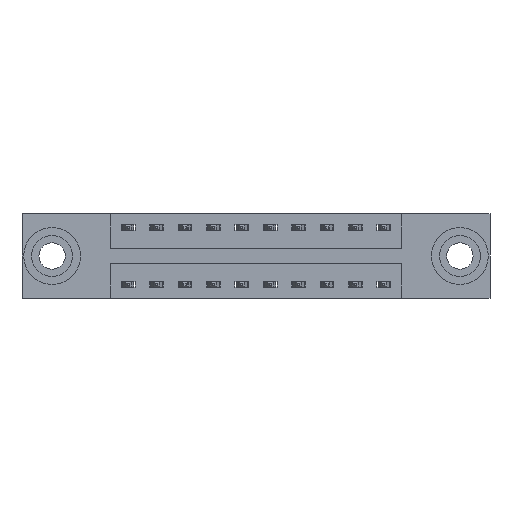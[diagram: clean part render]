
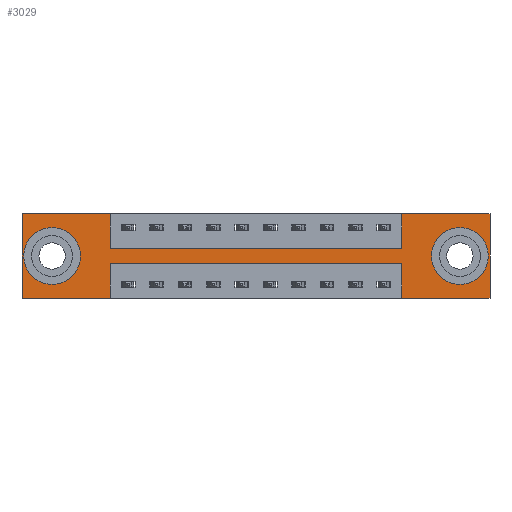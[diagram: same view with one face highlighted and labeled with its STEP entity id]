
A CAD part, front view. The second image highlights one B-rep face of the part: STEP entity #3029.
In plain terms, the highlighted planar face has unit normal (0, -1, 0).
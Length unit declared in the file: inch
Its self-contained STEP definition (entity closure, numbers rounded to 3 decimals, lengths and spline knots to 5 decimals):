
#283 = DIRECTION ( 'NONE',  ( 0., 0., -1. ) ) ;
#400 = DIRECTION ( 'NONE',  ( -1., 0., 0. ) ) ;
#418 = VERTEX_POINT ( 'NONE', #2137 ) ;
#450 = DIRECTION ( 'NONE',  ( 0., -1., 0. ) ) ;
#563 = VECTOR ( 'NONE', #8137, 39.37008 ) ;
#640 = CARTESIAN_POINT ( 'NONE',  ( 0., 0., -0.37 ) ) ;
#755 = LINE ( 'NONE', #9937, #563 ) ;
#928 = CARTESIAN_POINT ( 'NONE',  ( 0.1325, 0., -0.185 ) ) ;
#998 = ORIENTED_EDGE ( 'NONE', *, *, #1817, .F. ) ;
#1020 = ORIENTED_EDGE ( 'NONE', *, *, #8218, .F. ) ;
#1084 = ORIENTED_EDGE ( 'NONE', *, *, #1894, .F. ) ;
#1175 = VERTEX_POINT ( 'NONE', #8202 ) ;
#1240 = VERTEX_POINT ( 'NONE', #2220 ) ;
#1372 = EDGE_CURVE ( 'NONE', #11254, #5622, #755, .T. ) ;
#1417 = CARTESIAN_POINT ( 'NONE',  ( 0., 0., -0.37 ) ) ;
#1468 = DIRECTION ( 'NONE',  ( 1., 0., 0. ) ) ;
#1470 = CARTESIAN_POINT ( 'NONE',  ( 0., 0., -0.37 ) ) ;
#1503 = CARTESIAN_POINT ( 'NONE',  ( 0.1325, 0., -0.263 ) ) ;
#1510 = LINE ( 'NONE', #11668, #4019 ) ;
#1596 = EDGE_CURVE ( 'NONE', #10452, #1175, #2704, .T. ) ;
#1668 = CARTESIAN_POINT ( 'NONE',  ( 0., 0., 0. ) ) ;
#1709 = EDGE_LOOP ( 'NONE', ( #7760, #5570, #1020, #5582, #10190, #3095, #998, #7753, #9215, #1084, #11849, #6446 ) ) ;
#1753 = EDGE_CURVE ( 'NONE', #418, #9596, #5391, .T. ) ;
#1760 = CIRCLE ( 'NONE', #7940, 0.078 ) ;
#1817 = EDGE_CURVE ( 'NONE', #11834, #3620, #11511, .T. ) ;
#1894 = EDGE_CURVE ( 'NONE', #10943, #7213, #6140, .T. ) ;
#1963 = DIRECTION ( 'NONE',  ( 0., 0., 1. ) ) ;
#2026 = FACE_BOUND ( 'NONE', #10474, .T. ) ;
#2090 = CARTESIAN_POINT ( 'NONE',  ( 0., 0., 0. ) ) ;
#2137 = CARTESIAN_POINT ( 'NONE',  ( 1.9275, 0., -0.263 ) ) ;
#2142 = EDGE_CURVE ( 'NONE', #1240, #11254, #7917, .T. ) ;
#2166 = CARTESIAN_POINT ( 'NONE',  ( 1.6725, 0., -0.37 ) ) ;
#2220 = CARTESIAN_POINT ( 'NONE',  ( 1.6725, 0., -0.22 ) ) ;
#2416 = DIRECTION ( 'NONE',  ( 0., 1., 0. ) ) ;
#2452 = ORIENTED_EDGE ( 'NONE', *, *, #1753, .T. ) ;
#2470 = LINE ( 'NONE', #640, #4967 ) ;
#2604 = VERTEX_POINT ( 'NONE', #2166 ) ;
#2684 = VECTOR ( 'NONE', #8916, 39.37008 ) ;
#2704 = CIRCLE ( 'NONE', #7905, 0.078 ) ;
#2754 = EDGE_LOOP ( 'NONE', ( #5229, #2785 ) ) ;
#2785 = ORIENTED_EDGE ( 'NONE', *, *, #1596, .T. ) ;
#2808 = EDGE_CURVE ( 'NONE', #1175, #10452, #1760, .T. ) ;
#2999 = VERTEX_POINT ( 'NONE', #8491 ) ;
#3029 = ADVANCED_FACE ( 'NONE', ( #2026, #4878, #5725 ), #9387, .T. ) ;
#3070 = VECTOR ( 'NONE', #1468, 39.37008 ) ;
#3093 = DIRECTION ( 'NONE',  ( 1., 0., 0. ) ) ;
#3095 = ORIENTED_EDGE ( 'NONE', *, *, #10859, .F. ) ;
#3135 = DIRECTION ( 'NONE',  ( 0., 0., -1. ) ) ;
#3156 = EDGE_CURVE ( 'NONE', #5622, #8309, #3539, .T. ) ;
#3242 = DIRECTION ( 'NONE',  ( 0., 0., 1. ) ) ;
#3278 = VECTOR ( 'NONE', #7834, 39.37008 ) ;
#3320 = DIRECTION ( 'NONE',  ( 0., 0., 1. ) ) ;
#3539 = LINE ( 'NONE', #1470, #5500 ) ;
#3620 = VERTEX_POINT ( 'NONE', #11077 ) ;
#3794 = CARTESIAN_POINT ( 'NONE',  ( 0.3875, 0., 0. ) ) ;
#4019 = VECTOR ( 'NONE', #4307, 39.37008 ) ;
#4117 = LINE ( 'NONE', #11361, #5005 ) ;
#4129 = VECTOR ( 'NONE', #7740, 39.37008 ) ;
#4212 = DIRECTION ( 'NONE',  ( 0., 1., 0. ) ) ;
#4229 = CARTESIAN_POINT ( 'NONE',  ( 2.06, 0., 0. ) ) ;
#4307 = DIRECTION ( 'NONE',  ( 1., 0., 0. ) ) ;
#4337 = CARTESIAN_POINT ( 'NONE',  ( 0.1325, 0., -0.185 ) ) ;
#4403 = LINE ( 'NONE', #5307, #2684 ) ;
#4490 = ORIENTED_EDGE ( 'NONE', *, *, #4623, .T. ) ;
#4623 = EDGE_CURVE ( 'NONE', #9596, #418, #6674, .T. ) ;
#4627 = DIRECTION ( 'NONE',  ( 0., 1., 0. ) ) ;
#4681 = DIRECTION ( 'NONE',  ( 0., 0., -1. ) ) ;
#4878 = FACE_BOUND ( 'NONE', #2754, .T. ) ;
#4967 = VECTOR ( 'NONE', #400, 39.37008 ) ;
#5005 = VECTOR ( 'NONE', #3093, 39.37008 ) ;
#5229 = ORIENTED_EDGE ( 'NONE', *, *, #2808, .T. ) ;
#5252 = CARTESIAN_POINT ( 'NONE',  ( 1.9275, 0., -0.107 ) ) ;
#5307 = CARTESIAN_POINT ( 'NONE',  ( 2.06, 0., 0. ) ) ;
#5391 = CIRCLE ( 'NONE', #11591, 0.078 ) ;
#5478 = CARTESIAN_POINT ( 'NONE',  ( 1.9275, 0., -0.185 ) ) ;
#5500 = VECTOR ( 'NONE', #10606, 39.37008 ) ;
#5553 = VECTOR ( 'NONE', #1963, 39.37008 ) ;
#5570 = ORIENTED_EDGE ( 'NONE', *, *, #2142, .F. ) ;
#5582 = ORIENTED_EDGE ( 'NONE', *, *, #6201, .F. ) ;
#5622 = VERTEX_POINT ( 'NONE', #7486 ) ;
#5725 = FACE_OUTER_BOUND ( 'NONE', #1709, .T. ) ;
#5856 = LINE ( 'NONE', #2090, #3278 ) ;
#6140 = LINE ( 'NONE', #11684, #3070 ) ;
#6201 = EDGE_CURVE ( 'NONE', #2999, #2604, #2470, .T. ) ;
#6446 = ORIENTED_EDGE ( 'NONE', *, *, #3156, .F. ) ;
#6674 = CIRCLE ( 'NONE', #9938, 0.078 ) ;
#6825 = EDGE_CURVE ( 'NONE', #11154, #11834, #1510, .T. ) ;
#7213 = VERTEX_POINT ( 'NONE', #9839 ) ;
#7458 = LINE ( 'NONE', #11162, #5553 ) ;
#7486 = CARTESIAN_POINT ( 'NONE',  ( 0.3875, 0., -0.37 ) ) ;
#7740 = DIRECTION ( 'NONE',  ( -1., 0., 0. ) ) ;
#7753 = ORIENTED_EDGE ( 'NONE', *, *, #6825, .F. ) ;
#7760 = ORIENTED_EDGE ( 'NONE', *, *, #1372, .F. ) ;
#7834 = DIRECTION ( 'NONE',  ( 0., 0., 1. ) ) ;
#7905 = AXIS2_PLACEMENT_3D ( 'NONE', #928, #4627, #10173 ) ;
#7917 = LINE ( 'NONE', #10508, #4129 ) ;
#7940 = AXIS2_PLACEMENT_3D ( 'NONE', #4337, #2416, #3320 ) ;
#8072 = VECTOR ( 'NONE', #3242, 39.37008 ) ;
#8137 = DIRECTION ( 'NONE',  ( 0., 0., -1. ) ) ;
#8168 = EDGE_CURVE ( 'NONE', #7213, #11154, #10236, .T. ) ;
#8202 = CARTESIAN_POINT ( 'NONE',  ( 0.1325, 0., -0.107 ) ) ;
#8218 = EDGE_CURVE ( 'NONE', #2604, #1240, #7458, .T. ) ;
#8309 = VERTEX_POINT ( 'NONE', #1417 ) ;
#8363 = DIRECTION ( 'NONE',  ( 0., 1., 0. ) ) ;
#8491 = CARTESIAN_POINT ( 'NONE',  ( 2.06, 0., -0.37 ) ) ;
#8551 = CARTESIAN_POINT ( 'NONE',  ( 0., 0., -0.37 ) ) ;
#8871 = CARTESIAN_POINT ( 'NONE',  ( 1.6725, 0., -0.15 ) ) ;
#8916 = DIRECTION ( 'NONE',  ( 0., 0., -1. ) ) ;
#9150 = CARTESIAN_POINT ( 'NONE',  ( 0.3875, 0., -0.15 ) ) ;
#9215 = ORIENTED_EDGE ( 'NONE', *, *, #8168, .F. ) ;
#9387 = PLANE ( 'NONE',  #9546 ) ;
#9546 = AXIS2_PLACEMENT_3D ( 'NONE', #8551, #450, #283 ) ;
#9596 = VERTEX_POINT ( 'NONE', #5252 ) ;
#9687 = CARTESIAN_POINT ( 'NONE',  ( 1.9275, 0., -0.185 ) ) ;
#9839 = CARTESIAN_POINT ( 'NONE',  ( 0.3875, 0., 0. ) ) ;
#9937 = CARTESIAN_POINT ( 'NONE',  ( 0.3875, 0., -0.37 ) ) ;
#9938 = AXIS2_PLACEMENT_3D ( 'NONE', #5478, #8363, #4681 ) ;
#10173 = DIRECTION ( 'NONE',  ( 0., 0., 1. ) ) ;
#10190 = ORIENTED_EDGE ( 'NONE', *, *, #10972, .F. ) ;
#10236 = LINE ( 'NONE', #3794, #11344 ) ;
#10452 = VERTEX_POINT ( 'NONE', #1503 ) ;
#10474 = EDGE_LOOP ( 'NONE', ( #4490, #2452 ) ) ;
#10508 = CARTESIAN_POINT ( 'NONE',  ( 0.3875, 0., -0.22 ) ) ;
#10606 = DIRECTION ( 'NONE',  ( -1., 0., 0. ) ) ;
#10667 = CARTESIAN_POINT ( 'NONE',  ( 1.6725, 0., 0. ) ) ;
#10728 = DIRECTION ( 'NONE',  ( 0., 0., -1. ) ) ;
#10792 = VERTEX_POINT ( 'NONE', #4229 ) ;
#10859 = EDGE_CURVE ( 'NONE', #3620, #10792, #4117, .T. ) ;
#10943 = VERTEX_POINT ( 'NONE', #1668 ) ;
#10972 = EDGE_CURVE ( 'NONE', #10792, #2999, #4403, .T. ) ;
#11077 = CARTESIAN_POINT ( 'NONE',  ( 1.6725, 0., 0. ) ) ;
#11154 = VERTEX_POINT ( 'NONE', #9150 ) ;
#11162 = CARTESIAN_POINT ( 'NONE',  ( 1.6725, 0., -0.37 ) ) ;
#11254 = VERTEX_POINT ( 'NONE', #11402 ) ;
#11289 = EDGE_CURVE ( 'NONE', #8309, #10943, #5856, .T. ) ;
#11344 = VECTOR ( 'NONE', #3135, 39.37008 ) ;
#11361 = CARTESIAN_POINT ( 'NONE',  ( 0., 0., 0. ) ) ;
#11402 = CARTESIAN_POINT ( 'NONE',  ( 0.3875, 0., -0.22 ) ) ;
#11511 = LINE ( 'NONE', #10667, #8072 ) ;
#11591 = AXIS2_PLACEMENT_3D ( 'NONE', #9687, #4212, #10728 ) ;
#11668 = CARTESIAN_POINT ( 'NONE',  ( 0.3875, 0., -0.15 ) ) ;
#11684 = CARTESIAN_POINT ( 'NONE',  ( 0., 0., 0. ) ) ;
#11834 = VERTEX_POINT ( 'NONE', #8871 ) ;
#11849 = ORIENTED_EDGE ( 'NONE', *, *, #11289, .F. ) ;
